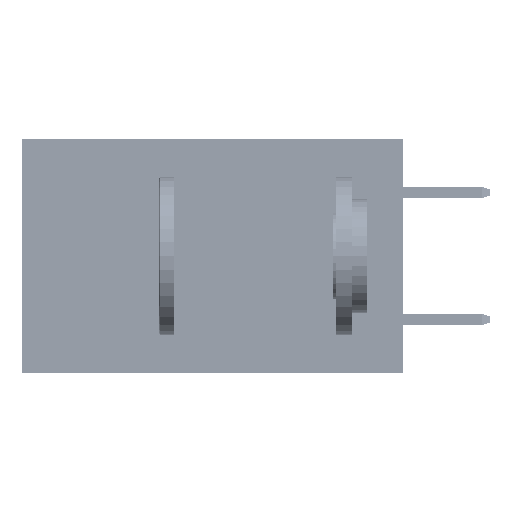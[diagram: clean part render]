
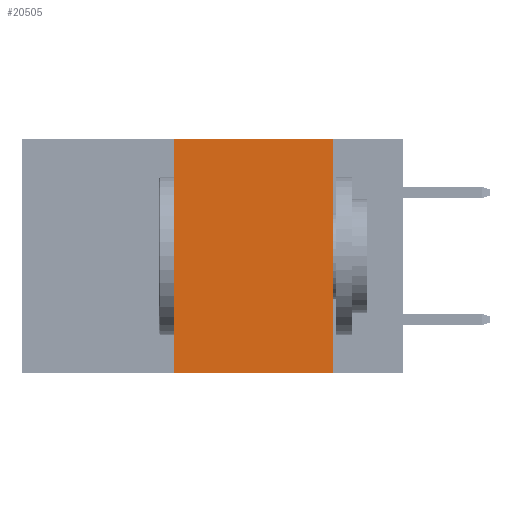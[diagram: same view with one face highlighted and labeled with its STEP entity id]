
A CAD part, left-side view. The second image highlights one B-rep face of the part: STEP entity #20505.
In plain terms, the highlighted planar face has unit normal (-1, 0, 0).
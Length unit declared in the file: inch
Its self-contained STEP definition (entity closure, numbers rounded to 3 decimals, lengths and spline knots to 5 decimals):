
#853 = VERTEX_POINT ( 'NONE', #44245 ) ;
#2219 = EDGE_CURVE ( 'NONE', #49434, #21879, #17490, .T. ) ;
#3429 = ORIENTED_EDGE ( 'NONE', *, *, #26251, .F. ) ;
#6049 = CARTESIAN_POINT ( 'NONE',  ( 0., 0.6, 0. ) ) ;
#7214 = CARTESIAN_POINT ( 'NONE',  ( 0., 0.36, -0.37 ) ) ;
#8408 = LINE ( 'NONE', #43198, #23657 ) ;
#9820 = PLANE ( 'NONE',  #35930 ) ;
#10212 = EDGE_CURVE ( 'NONE', #49434, #853, #8408, .T. ) ;
#10462 = CARTESIAN_POINT ( 'NONE',  ( 0., 0.6, -0.37 ) ) ;
#10738 = EDGE_CURVE ( 'NONE', #42713, #21879, #26863, .T. ) ;
#12921 = CARTESIAN_POINT ( 'NONE',  ( 0., 0.11, 0. ) ) ;
#16470 = CARTESIAN_POINT ( 'NONE',  ( 0., 0.6, 0. ) ) ;
#17087 = DIRECTION ( 'NONE',  ( 1., 0., 0. ) ) ;
#17490 = LINE ( 'NONE', #10462, #32468 ) ;
#19371 = DIRECTION ( 'NONE',  ( 0., 0., -1. ) ) ;
#20505 = ADVANCED_FACE ( 'NONE', ( #44094 ), #9820, .F. ) ;
#21879 = VERTEX_POINT ( 'NONE', #26537 ) ;
#22278 = EDGE_LOOP ( 'NONE', ( #47587, #3429, #42246, #38944 ) ) ;
#23657 = VECTOR ( 'NONE', #35424, 39.37008 ) ;
#23696 = VECTOR ( 'NONE', #19371, 39.37008 ) ;
#24468 = LINE ( 'NONE', #16470, #37806 ) ;
#24585 = DIRECTION ( 'NONE',  ( 0., 0., -1. ) ) ;
#26251 = EDGE_CURVE ( 'NONE', #853, #42713, #24468, .T. ) ;
#26537 = CARTESIAN_POINT ( 'NONE',  ( 0., 0.11, -0.37 ) ) ;
#26863 = LINE ( 'NONE', #43141, #23696 ) ;
#31727 = DIRECTION ( 'NONE',  ( 0., -1., 0. ) ) ;
#32468 = VECTOR ( 'NONE', #44496, 39.37008 ) ;
#35424 = DIRECTION ( 'NONE',  ( 0., 0., 1. ) ) ;
#35930 = AXIS2_PLACEMENT_3D ( 'NONE', #6049, #17087, #24585 ) ;
#37806 = VECTOR ( 'NONE', #31727, 39.37008 ) ;
#38944 = ORIENTED_EDGE ( 'NONE', *, *, #2219, .T. ) ;
#42246 = ORIENTED_EDGE ( 'NONE', *, *, #10212, .F. ) ;
#42713 = VERTEX_POINT ( 'NONE', #12921 ) ;
#43141 = CARTESIAN_POINT ( 'NONE',  ( 0., 0.11, 0. ) ) ;
#43198 = CARTESIAN_POINT ( 'NONE',  ( 0., 0.36, 0. ) ) ;
#44094 = FACE_OUTER_BOUND ( 'NONE', #22278, .T. ) ;
#44245 = CARTESIAN_POINT ( 'NONE',  ( 0., 0.36, 0. ) ) ;
#44496 = DIRECTION ( 'NONE',  ( 0., -1., 0. ) ) ;
#47587 = ORIENTED_EDGE ( 'NONE', *, *, #10738, .F. ) ;
#49434 = VERTEX_POINT ( 'NONE', #7214 ) ;
